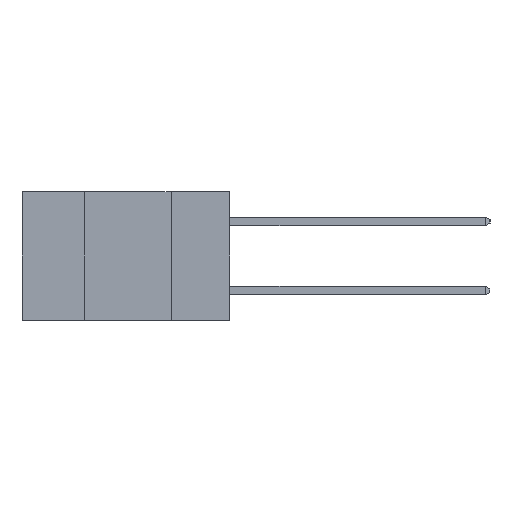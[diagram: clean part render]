
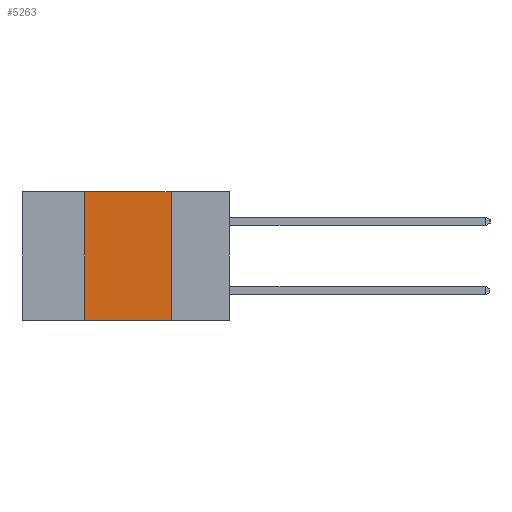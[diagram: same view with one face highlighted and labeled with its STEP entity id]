
A CAD part, left-side view. The second image highlights one B-rep face of the part: STEP entity #5263.
In plain terms, the highlighted planar face has unit normal (-1, 0, 0).
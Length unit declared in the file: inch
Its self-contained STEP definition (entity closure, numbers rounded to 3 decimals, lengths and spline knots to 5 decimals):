
#104 = ORIENTED_EDGE ( 'NONE', *, *, #11063, .F. ) ;
#375 = VERTEX_POINT ( 'NONE', #6098 ) ;
#427 = CARTESIAN_POINT ( 'NONE',  ( 0., 0.17, 0. ) ) ;
#715 = DIRECTION ( 'NONE',  ( 0., 0., -1. ) ) ;
#760 = CARTESIAN_POINT ( 'NONE',  ( 0., 0.17, -0.37 ) ) ;
#2069 = LINE ( 'NONE', #2087, #9948 ) ;
#2087 = CARTESIAN_POINT ( 'NONE',  ( 0., 0.42, 0. ) ) ;
#2746 = VECTOR ( 'NONE', #5421, 39.37008 ) ;
#2904 = EDGE_LOOP ( 'NONE', ( #10057, #104, #10817, #6170 ) ) ;
#4628 = AXIS2_PLACEMENT_3D ( 'NONE', #5413, #7528, #715 ) ;
#5263 = ADVANCED_FACE ( 'NONE', ( #5717 ), #10435, .F. ) ;
#5284 = EDGE_CURVE ( 'NONE', #8029, #12088, #9055, .T. ) ;
#5413 = CARTESIAN_POINT ( 'NONE',  ( 0., 0.6, 0. ) ) ;
#5421 = DIRECTION ( 'NONE',  ( 0., -1., 0. ) ) ;
#5428 = LINE ( 'NONE', #11404, #2746 ) ;
#5705 = LINE ( 'NONE', #11020, #10718 ) ;
#5717 = FACE_OUTER_BOUND ( 'NONE', #2904, .T. ) ;
#5759 = EDGE_CURVE ( 'NONE', #9624, #12088, #5705, .T. ) ;
#6094 = EDGE_CURVE ( 'NONE', #9624, #375, #2069, .T. ) ;
#6098 = CARTESIAN_POINT ( 'NONE',  ( 0., 0.42, 0. ) ) ;
#6170 = ORIENTED_EDGE ( 'NONE', *, *, #5759, .T. ) ;
#7528 = DIRECTION ( 'NONE',  ( 1., 0., 0. ) ) ;
#7646 = DIRECTION ( 'NONE',  ( 0., 0., 1. ) ) ;
#8029 = VERTEX_POINT ( 'NONE', #427 ) ;
#8179 = DIRECTION ( 'NONE',  ( 0., -1., 0. ) ) ;
#9055 = LINE ( 'NONE', #12391, #13246 ) ;
#9624 = VERTEX_POINT ( 'NONE', #12879 ) ;
#9948 = VECTOR ( 'NONE', #7646, 39.37008 ) ;
#10057 = ORIENTED_EDGE ( 'NONE', *, *, #5284, .F. ) ;
#10435 = PLANE ( 'NONE',  #4628 ) ;
#10718 = VECTOR ( 'NONE', #8179, 39.37008 ) ;
#10817 = ORIENTED_EDGE ( 'NONE', *, *, #6094, .F. ) ;
#11020 = CARTESIAN_POINT ( 'NONE',  ( 0., 0.6, -0.37 ) ) ;
#11063 = EDGE_CURVE ( 'NONE', #375, #8029, #5428, .T. ) ;
#11404 = CARTESIAN_POINT ( 'NONE',  ( 0., 0.6, 0. ) ) ;
#12088 = VERTEX_POINT ( 'NONE', #760 ) ;
#12391 = CARTESIAN_POINT ( 'NONE',  ( 0., 0.17, 0. ) ) ;
#12879 = CARTESIAN_POINT ( 'NONE',  ( 0., 0.42, -0.37 ) ) ;
#13246 = VECTOR ( 'NONE', #13338, 39.37008 ) ;
#13338 = DIRECTION ( 'NONE',  ( 0., 0., -1. ) ) ;
